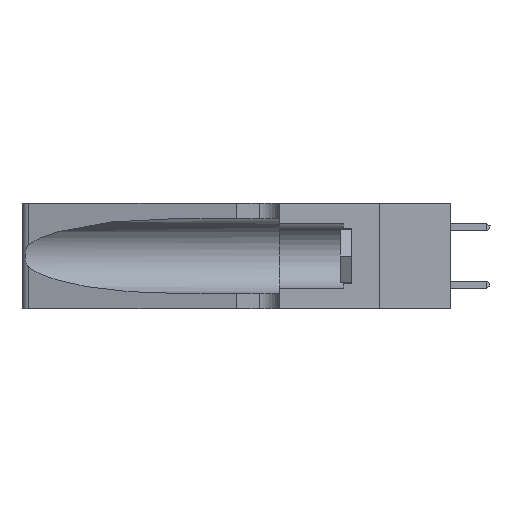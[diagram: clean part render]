
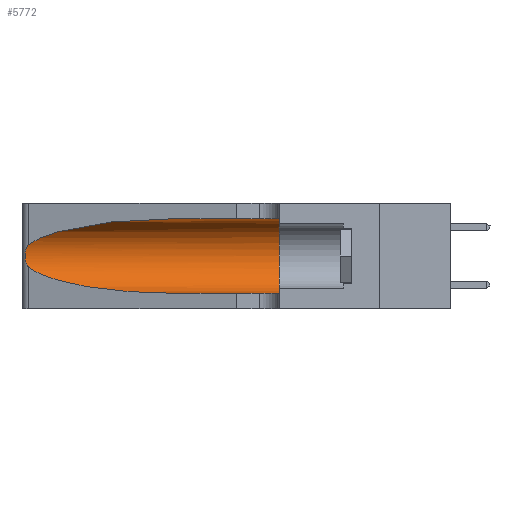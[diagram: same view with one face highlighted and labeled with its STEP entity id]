
A CAD part, left-side view. The second image highlights one B-rep face of the part: STEP entity #5772.
In plain terms, the highlighted cylindrical face has radius 3.308 mm (diameter 6.617 mm), a partial arc.
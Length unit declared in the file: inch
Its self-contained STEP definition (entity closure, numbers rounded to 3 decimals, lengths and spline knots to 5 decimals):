
#217 = CARTESIAN_POINT ( 'NONE',  ( 0.1305, 0.35, 0.05475 ) ) ;
#735 = CARTESIAN_POINT ( 'NONE',  ( 0.2373, 1.15595, 0.08982 ) ) ;
#761 = B_SPLINE_CURVE_WITH_KNOTS ( 'NONE', 3,
 ( #10199, #2602, #13889, #2686, #15732, #4631, #17564, #6547, #19379, #8431, #21202, #10285, #23055, #12151 ),
 .UNSPECIFIED., .F., .F.,
 ( 4, 2, 2, 2, 2, 2, 4 ),
 ( 0., 0.00027, 0.00053, 0.00107, 0.0016, 0.00187, 0.00214 ),
 .UNSPECIFIED. ) ;
#1863 = CARTESIAN_POINT ( 'NONE',  ( 0.1305, 0.35, 0.185 ) ) ;
#2115 = ORIENTED_EDGE ( 'NONE', *, *, #15228, .T. ) ;
#2189 = CIRCLE ( 'NONE', #7023, 0.13025 ) ;
#2602 = CARTESIAN_POINT ( 'NONE',  ( 0.25555, 1.22994, 0.2215 ) ) ;
#2686 = CARTESIAN_POINT ( 'NONE',  ( 0.25787, 1.23484, 0.2124 ) ) ;
#2881 = VERTEX_POINT ( 'NONE', #20949 ) ;
#3813 = DIRECTION ( 'NONE',  ( 0., 0., 1. ) ) ;
#4495 = EDGE_CURVE ( 'NONE', #19763, #6169, #17047, .T. ) ;
#4631 = CARTESIAN_POINT ( 'NONE',  ( 0.26018, 1.23835, 0.19895 ) ) ;
#4706 = CARTESIAN_POINT ( 'NONE',  ( 0.1305, 0.72297, 0.05475 ) ) ;
#5092 = FACE_OUTER_BOUND ( 'NONE', #23818, .T. ) ;
#5634 = CARTESIAN_POINT ( 'NONE',  ( 0.1305, 1.61858, 0.31525 ) ) ;
#5714 = DIRECTION ( 'NONE',  ( 0., -1., 0. ) ) ;
#5746 = VECTOR ( 'NONE', #5714, 39.37008 ) ;
#5772 = ADVANCED_FACE ( 'NONE', ( #5092 ), #14384, .F. ) ;
#6169 = VERTEX_POINT ( 'NONE', #217 ) ;
#6341 = CARTESIAN_POINT ( 'NONE',  ( 0.2373, 1.15595, 0.28018 ) ) ;
#6547 = CARTESIAN_POINT ( 'NONE',  ( 0.26075, 1.23896, 0.178 ) ) ;
#6947 = LINE ( 'NONE', #5634, #5746 ) ;
#7023 = AXIS2_PLACEMENT_3D ( 'NONE', #1863, #14933, #3813 ) ;
#7271 = VECTOR ( 'NONE', #8737, 39.37008 ) ;
#7331 = ORIENTED_EDGE ( 'NONE', *, *, #22690, .F. ) ;
#8009 = CARTESIAN_POINT ( 'NONE',  ( 0.1305, 0.72297, 0.31525 ) ) ;
#8431 = CARTESIAN_POINT ( 'NONE',  ( 0.25856, 1.23593, 0.16098 ) ) ;
#8737 = DIRECTION ( 'NONE',  ( 0., -1., 0. ) ) ;
#8765 = ORIENTED_EDGE ( 'NONE', *, *, #20555, .T. ) ;
#8777 = VERTEX_POINT ( 'NONE', #8009 ) ;
#9604 =( BOUNDED_CURVE ( )  B_SPLINE_CURVE ( 3, ( #15536, #17377, #6341, #19185 ),
 .UNSPECIFIED., .F., .F. ) 
 B_SPLINE_CURVE_WITH_KNOTS ( ( 4, 4 ),
 ( 1.5708, 2.84003 ),
 .UNSPECIFIED. ) 
 CURVE ( )  GEOMETRIC_REPRESENTATION_ITEM ( )  RATIONAL_B_SPLINE_CURVE ( ( 1., 0.87, 0.87, 1. ) ) 
 REPRESENTATION_ITEM ( '' )  );
#10199 = CARTESIAN_POINT ( 'NONE',  ( 0.25487, 1.22718, 0.22369 ) ) ;
#10285 = CARTESIAN_POINT ( 'NONE',  ( 0.25639, 1.23186, 0.15144 ) ) ;
#12151 = CARTESIAN_POINT ( 'NONE',  ( 0.25487, 1.22718, 0.14631 ) ) ;
#12371 = CARTESIAN_POINT ( 'NONE',  ( 0.1305, 1.61858, 0.05475 ) ) ;
#12907 = CARTESIAN_POINT ( 'NONE',  ( 0.25487, 1.22718, 0.22369 ) ) ;
#13700 = CARTESIAN_POINT ( 'NONE',  ( 0.1305, 0.72297, 0.05475 ) ) ;
#13889 = CARTESIAN_POINT ( 'NONE',  ( 0.25639, 1.23184, 0.21858 ) ) ;
#14208 = ORIENTED_EDGE ( 'NONE', *, *, #21981, .F. ) ;
#14384 = CYLINDRICAL_SURFACE ( 'NONE', #17341, 0.13025 ) ;
#14834 = ORIENTED_EDGE ( 'NONE', *, *, #20556, .T. ) ;
#14933 = DIRECTION ( 'NONE',  ( 0., 1., 0. ) ) ;
#15228 = EDGE_CURVE ( 'NONE', #8777, #18579, #9604, .T. ) ;
#15536 = CARTESIAN_POINT ( 'NONE',  ( 0.1305, 0.72297, 0.31525 ) ) ;
#15732 = CARTESIAN_POINT ( 'NONE',  ( 0.25854, 1.2359, 0.20912 ) ) ;
#15810 = CARTESIAN_POINT ( 'NONE',  ( 0.18966, 0.96281, 0.05475 ) ) ;
#17047 = LINE ( 'NONE', #12371, #7271 ) ;
#17341 = AXIS2_PLACEMENT_3D ( 'NONE', #21469, #17833, #21392 ) ;
#17377 = CARTESIAN_POINT ( 'NONE',  ( 0.18966, 0.96281, 0.31525 ) ) ;
#17564 = CARTESIAN_POINT ( 'NONE',  ( 0.26075, 1.23896, 0.19203 ) ) ;
#17606 = VERTEX_POINT ( 'NONE', #19237 ) ;
#17833 = DIRECTION ( 'NONE',  ( 0., -1., 0. ) ) ;
#18579 = VERTEX_POINT ( 'NONE', #12907 ) ;
#19185 = CARTESIAN_POINT ( 'NONE',  ( 0.25487, 1.22718, 0.22369 ) ) ;
#19237 = CARTESIAN_POINT ( 'NONE',  ( 0.1305, 0.35, 0.31525 ) ) ;
#19379 = CARTESIAN_POINT ( 'NONE',  ( 0.26017, 1.23833, 0.17102 ) ) ;
#19645 = ORIENTED_EDGE ( 'NONE', *, *, #4495, .T. ) ;
#19763 = VERTEX_POINT ( 'NONE', #13700 ) ;
#20555 = EDGE_CURVE ( 'NONE', #18579, #2881, #761, .T. ) ;
#20556 = EDGE_CURVE ( 'NONE', #2881, #19763, #20579, .T. ) ;
#20579 =( BOUNDED_CURVE ( )  B_SPLINE_CURVE ( 3, ( #22970, #735, #15810, #4706 ),
 .UNSPECIFIED., .F., .F. ) 
 B_SPLINE_CURVE_WITH_KNOTS ( ( 4, 4 ),
 ( 3.44316, 4.71239 ),
 .UNSPECIFIED. ) 
 CURVE ( )  GEOMETRIC_REPRESENTATION_ITEM ( )  RATIONAL_B_SPLINE_CURVE ( ( 1., 0.87, 0.87, 1. ) ) 
 REPRESENTATION_ITEM ( '' )  );
#20949 = CARTESIAN_POINT ( 'NONE',  ( 0.25487, 1.22718, 0.14631 ) ) ;
#21202 = CARTESIAN_POINT ( 'NONE',  ( 0.25789, 1.23486, 0.15765 ) ) ;
#21392 = DIRECTION ( 'NONE',  ( 0., 0., -1. ) ) ;
#21469 = CARTESIAN_POINT ( 'NONE',  ( 0.1305, 1.61858, 0.185 ) ) ;
#21981 = EDGE_CURVE ( 'NONE', #17606, #6169, #2189, .T. ) ;
#22690 = EDGE_CURVE ( 'NONE', #8777, #17606, #6947, .T. ) ;
#22970 = CARTESIAN_POINT ( 'NONE',  ( 0.25487, 1.22718, 0.14631 ) ) ;
#23055 = CARTESIAN_POINT ( 'NONE',  ( 0.25555, 1.22993, 0.14849 ) ) ;
#23818 = EDGE_LOOP ( 'NONE', ( #2115, #8765, #14834, #19645, #14208, #7331 ) ) ;
